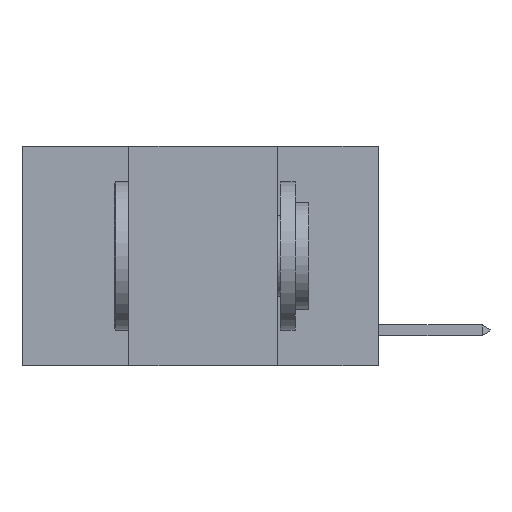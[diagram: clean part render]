
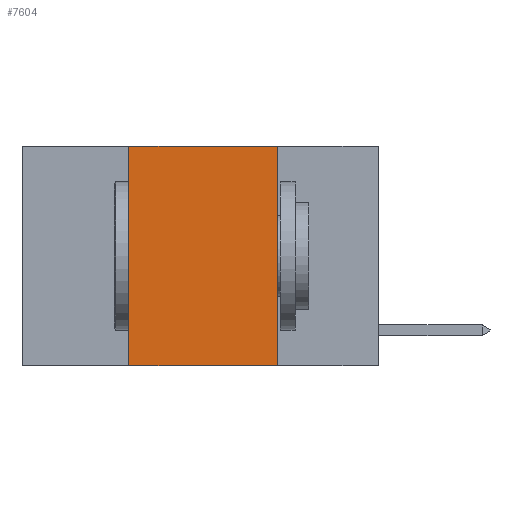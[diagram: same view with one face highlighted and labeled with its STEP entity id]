
A CAD part, left-side view. The second image highlights one B-rep face of the part: STEP entity #7604.
In plain terms, the highlighted planar face has unit normal (-1, 0, 0).
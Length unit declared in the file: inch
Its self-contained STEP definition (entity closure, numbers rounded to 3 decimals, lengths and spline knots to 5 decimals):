
#60 = CARTESIAN_POINT ( 'NONE',  ( 0., 0.6, -0.37 ) ) ;
#343 = DIRECTION ( 'NONE',  ( 0., -1., 0. ) ) ;
#1063 = VERTEX_POINT ( 'NONE', #13544 ) ;
#2328 = CARTESIAN_POINT ( 'NONE',  ( 0., 0.42, -0.37 ) ) ;
#2678 = CARTESIAN_POINT ( 'NONE',  ( 0., 0.6, 0. ) ) ;
#3176 = PLANE ( 'NONE',  #17632 ) ;
#3814 = VECTOR ( 'NONE', #19208, 39.37008 ) ;
#4800 = CARTESIAN_POINT ( 'NONE',  ( 0., 0.17, 0. ) ) ;
#5353 = ORIENTED_EDGE ( 'NONE', *, *, #19876, .F. ) ;
#7604 = ADVANCED_FACE ( 'NONE', ( #21179 ), #3176, .F. ) ;
#7969 = VECTOR ( 'NONE', #22310, 39.37008 ) ;
#9729 = CARTESIAN_POINT ( 'NONE',  ( 0., 0.6, 0. ) ) ;
#9999 = EDGE_CURVE ( 'NONE', #13195, #26714, #16142, .T. ) ;
#10485 = EDGE_CURVE ( 'NONE', #26714, #1063, #10779, .T. ) ;
#10756 = ORIENTED_EDGE ( 'NONE', *, *, #9999, .F. ) ;
#10779 = LINE ( 'NONE', #4800, #3814 ) ;
#12878 = CARTESIAN_POINT ( 'NONE',  ( 0., 0.42, 0. ) ) ;
#13076 = VECTOR ( 'NONE', #343, 39.37008 ) ;
#13195 = VERTEX_POINT ( 'NONE', #12878 ) ;
#13544 = CARTESIAN_POINT ( 'NONE',  ( 0., 0.17, -0.37 ) ) ;
#14731 = EDGE_CURVE ( 'NONE', #23145, #1063, #24987, .T. ) ;
#16142 = LINE ( 'NONE', #9729, #26383 ) ;
#17632 = AXIS2_PLACEMENT_3D ( 'NONE', #2678, #23228, #21811 ) ;
#18011 = ORIENTED_EDGE ( 'NONE', *, *, #10485, .F. ) ;
#18085 = CARTESIAN_POINT ( 'NONE',  ( 0., 0.42, 0. ) ) ;
#19208 = DIRECTION ( 'NONE',  ( 0., 0., -1. ) ) ;
#19876 = EDGE_CURVE ( 'NONE', #23145, #13195, #26832, .T. ) ;
#21179 = FACE_OUTER_BOUND ( 'NONE', #24891, .T. ) ;
#21811 = DIRECTION ( 'NONE',  ( 0., 0., -1. ) ) ;
#22274 = DIRECTION ( 'NONE',  ( 0., -1., 0. ) ) ;
#22310 = DIRECTION ( 'NONE',  ( 0., 0., 1. ) ) ;
#23139 = CARTESIAN_POINT ( 'NONE',  ( 0., 0.17, 0. ) ) ;
#23145 = VERTEX_POINT ( 'NONE', #2328 ) ;
#23228 = DIRECTION ( 'NONE',  ( 1., 0., 0. ) ) ;
#24891 = EDGE_LOOP ( 'NONE', ( #18011, #10756, #5353, #25544 ) ) ;
#24987 = LINE ( 'NONE', #60, #13076 ) ;
#25544 = ORIENTED_EDGE ( 'NONE', *, *, #14731, .T. ) ;
#26383 = VECTOR ( 'NONE', #22274, 39.37008 ) ;
#26714 = VERTEX_POINT ( 'NONE', #23139 ) ;
#26832 = LINE ( 'NONE', #18085, #7969 ) ;
